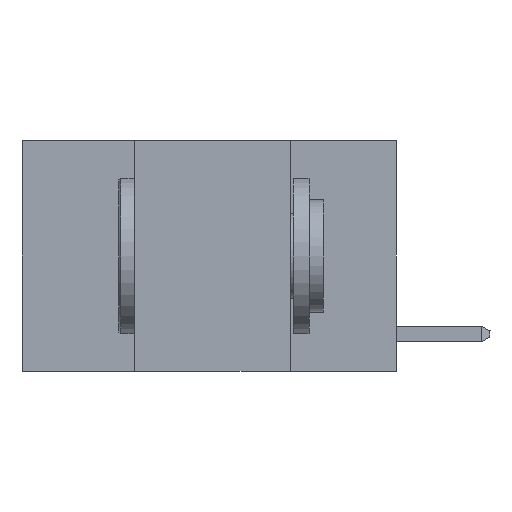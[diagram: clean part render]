
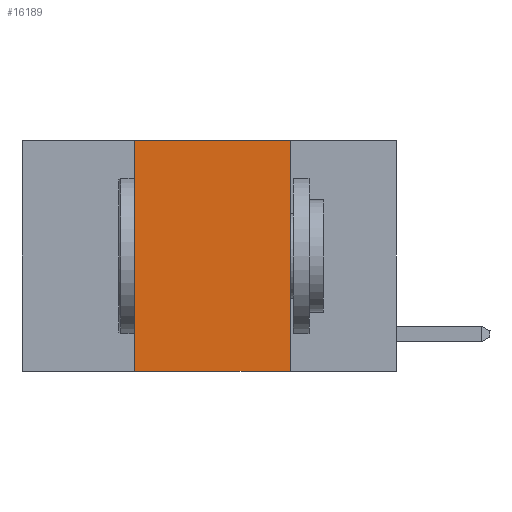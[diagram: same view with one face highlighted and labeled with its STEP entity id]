
A CAD part, left-side view. The second image highlights one B-rep face of the part: STEP entity #16189.
In plain terms, the highlighted planar face has unit normal (-1, 0, 0).
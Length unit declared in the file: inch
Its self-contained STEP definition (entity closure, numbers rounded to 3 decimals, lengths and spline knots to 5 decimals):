
#628 = VERTEX_POINT ( 'NONE', #25076 ) ;
#838 = CARTESIAN_POINT ( 'NONE',  ( 0., 0.6, 0. ) ) ;
#1173 = VECTOR ( 'NONE', #19087, 39.37008 ) ;
#1232 = ORIENTED_EDGE ( 'NONE', *, *, #15404, .F. ) ;
#5986 = LINE ( 'NONE', #10557, #17748 ) ;
#6068 = DIRECTION ( 'NONE',  ( 0., 0., -1. ) ) ;
#7400 = CARTESIAN_POINT ( 'NONE',  ( 0., 0.6, -0.37 ) ) ;
#7565 = CARTESIAN_POINT ( 'NONE',  ( 0., 0.17, 0. ) ) ;
#7965 = DIRECTION ( 'NONE',  ( 1., 0., 0. ) ) ;
#8276 = PLANE ( 'NONE',  #28351 ) ;
#8590 = FACE_OUTER_BOUND ( 'NONE', #9157, .T. ) ;
#9157 = EDGE_LOOP ( 'NONE', ( #30108, #1232, #20860, #25286 ) ) ;
#10557 = CARTESIAN_POINT ( 'NONE',  ( 0., 0.6, 0. ) ) ;
#12010 = VERTEX_POINT ( 'NONE', #25472 ) ;
#12470 = VERTEX_POINT ( 'NONE', #7565 ) ;
#12671 = VERTEX_POINT ( 'NONE', #22864 ) ;
#14582 = CARTESIAN_POINT ( 'NONE',  ( 0., 0.17, 0. ) ) ;
#14735 = EDGE_CURVE ( 'NONE', #12470, #12010, #16971, .T. ) ;
#15404 = EDGE_CURVE ( 'NONE', #628, #12470, #5986, .T. ) ;
#16189 = ADVANCED_FACE ( 'NONE', ( #8590 ), #8276, .F. ) ;
#16971 = LINE ( 'NONE', #14582, #26781 ) ;
#16982 = EDGE_CURVE ( 'NONE', #12671, #628, #19548, .T. ) ;
#17748 = VECTOR ( 'NONE', #29788, 39.37008 ) ;
#19087 = DIRECTION ( 'NONE',  ( 0., 0., 1. ) ) ;
#19548 = LINE ( 'NONE', #26171, #1173 ) ;
#20860 = ORIENTED_EDGE ( 'NONE', *, *, #16982, .F. ) ;
#22864 = CARTESIAN_POINT ( 'NONE',  ( 0., 0.42, -0.37 ) ) ;
#23914 = DIRECTION ( 'NONE',  ( 0., 0., -1. ) ) ;
#24777 = VECTOR ( 'NONE', #26500, 39.37008 ) ;
#25076 = CARTESIAN_POINT ( 'NONE',  ( 0., 0.42, 0. ) ) ;
#25286 = ORIENTED_EDGE ( 'NONE', *, *, #30447, .T. ) ;
#25472 = CARTESIAN_POINT ( 'NONE',  ( 0., 0.17, -0.37 ) ) ;
#26171 = CARTESIAN_POINT ( 'NONE',  ( 0., 0.42, 0. ) ) ;
#26500 = DIRECTION ( 'NONE',  ( 0., -1., 0. ) ) ;
#26781 = VECTOR ( 'NONE', #23914, 39.37008 ) ;
#28351 = AXIS2_PLACEMENT_3D ( 'NONE', #838, #7965, #6068 ) ;
#29147 = LINE ( 'NONE', #7400, #24777 ) ;
#29788 = DIRECTION ( 'NONE',  ( 0., -1., 0. ) ) ;
#30108 = ORIENTED_EDGE ( 'NONE', *, *, #14735, .F. ) ;
#30447 = EDGE_CURVE ( 'NONE', #12671, #12010, #29147, .T. ) ;
